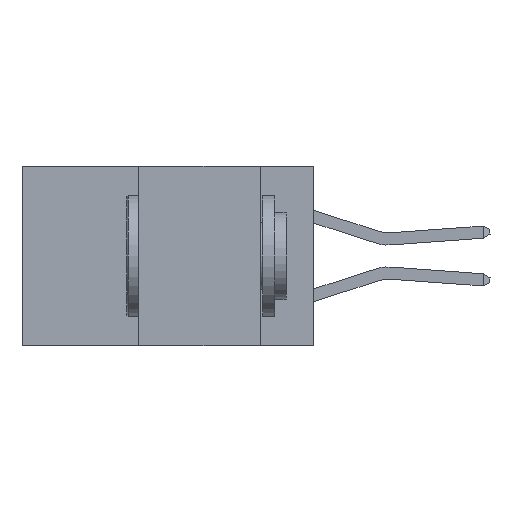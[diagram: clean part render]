
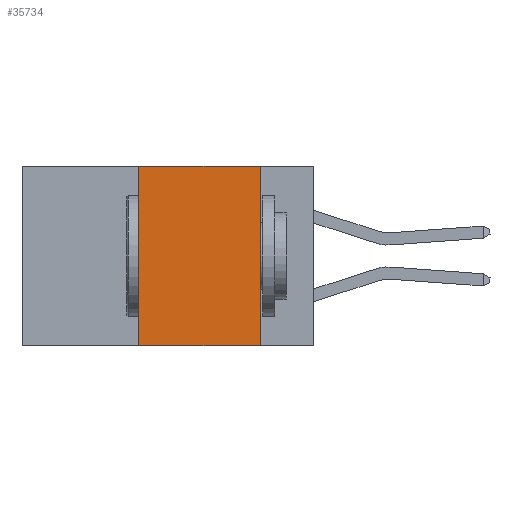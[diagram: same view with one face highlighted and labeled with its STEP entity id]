
A CAD part, left-side view. The second image highlights one B-rep face of the part: STEP entity #35734.
In plain terms, the highlighted planar face has unit normal (-1, 0, 0).
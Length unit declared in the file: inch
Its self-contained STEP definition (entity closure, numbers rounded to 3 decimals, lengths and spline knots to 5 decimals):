
#1316 = ORIENTED_EDGE ( 'NONE', *, *, #22690, .T. ) ;
#3519 = EDGE_CURVE ( 'NONE', #20645, #9889, #10745, .T. ) ;
#4383 = VERTEX_POINT ( 'NONE', #36754 ) ;
#5250 = CARTESIAN_POINT ( 'NONE',  ( 0., 0.36, 0. ) ) ;
#5274 = VECTOR ( 'NONE', #24147, 39.37008 ) ;
#6560 = EDGE_CURVE ( 'NONE', #9889, #4383, #25159, .T. ) ;
#6798 = CARTESIAN_POINT ( 'NONE',  ( 0., 0.11, 0. ) ) ;
#9395 = VERTEX_POINT ( 'NONE', #29555 ) ;
#9889 = VERTEX_POINT ( 'NONE', #6798 ) ;
#10288 = EDGE_CURVE ( 'NONE', #9395, #20645, #13922, .T. ) ;
#10745 = LINE ( 'NONE', #14660, #19826 ) ;
#11892 = DIRECTION ( 'NONE',  ( 1., 0., 0. ) ) ;
#12132 = CARTESIAN_POINT ( 'NONE',  ( 0., 0.36, 0. ) ) ;
#12262 = VECTOR ( 'NONE', #27332, 39.37008 ) ;
#13025 = FACE_OUTER_BOUND ( 'NONE', #24392, .T. ) ;
#13046 = AXIS2_PLACEMENT_3D ( 'NONE', #38609, #11892, #24423 ) ;
#13922 = LINE ( 'NONE', #12132, #5274 ) ;
#14660 = CARTESIAN_POINT ( 'NONE',  ( 0., 0.6, 0. ) ) ;
#15588 = LINE ( 'NONE', #20815, #12262 ) ;
#17625 = ORIENTED_EDGE ( 'NONE', *, *, #6560, .F. ) ;
#17991 = ORIENTED_EDGE ( 'NONE', *, *, #10288, .F. ) ;
#19815 = DIRECTION ( 'NONE',  ( 0., 0., -1. ) ) ;
#19826 = VECTOR ( 'NONE', #32760, 39.37008 ) ;
#20645 = VERTEX_POINT ( 'NONE', #5250 ) ;
#20815 = CARTESIAN_POINT ( 'NONE',  ( 0., 0.6, -0.37 ) ) ;
#22203 = ORIENTED_EDGE ( 'NONE', *, *, #3519, .F. ) ;
#22690 = EDGE_CURVE ( 'NONE', #9395, #4383, #15588, .T. ) ;
#24147 = DIRECTION ( 'NONE',  ( 0., 0., 1. ) ) ;
#24392 = EDGE_LOOP ( 'NONE', ( #17625, #22203, #17991, #1316 ) ) ;
#24423 = DIRECTION ( 'NONE',  ( 0., 0., -1. ) ) ;
#25159 = LINE ( 'NONE', #38076, #27056 ) ;
#27056 = VECTOR ( 'NONE', #19815, 39.37008 ) ;
#27332 = DIRECTION ( 'NONE',  ( 0., -1., 0. ) ) ;
#29555 = CARTESIAN_POINT ( 'NONE',  ( 0., 0.36, -0.37 ) ) ;
#32760 = DIRECTION ( 'NONE',  ( 0., -1., 0. ) ) ;
#35533 = PLANE ( 'NONE',  #13046 ) ;
#35734 = ADVANCED_FACE ( 'NONE', ( #13025 ), #35533, .F. ) ;
#36754 = CARTESIAN_POINT ( 'NONE',  ( 0., 0.11, -0.37 ) ) ;
#38076 = CARTESIAN_POINT ( 'NONE',  ( 0., 0.11, 0. ) ) ;
#38609 = CARTESIAN_POINT ( 'NONE',  ( 0., 0.6, 0. ) ) ;
